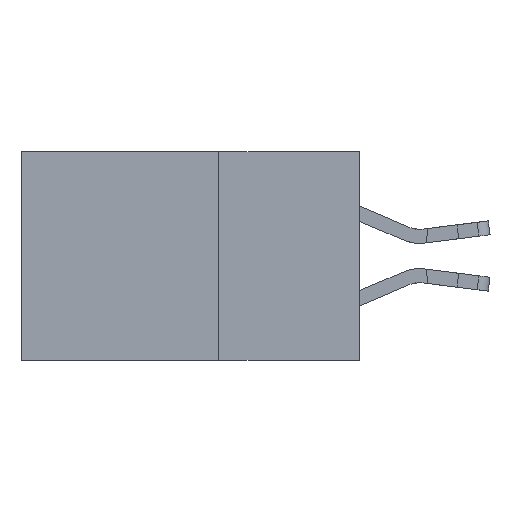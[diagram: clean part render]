
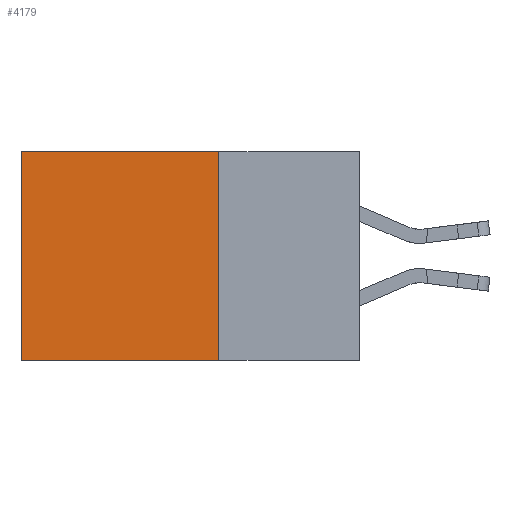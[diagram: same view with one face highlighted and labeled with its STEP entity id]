
A CAD part, left-side view. The second image highlights one B-rep face of the part: STEP entity #4179.
In plain terms, the highlighted planar face has unit normal (-1, 0, 0).
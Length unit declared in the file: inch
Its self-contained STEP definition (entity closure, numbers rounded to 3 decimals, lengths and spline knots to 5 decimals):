
#1412 = CARTESIAN_POINT ( 'NONE',  ( 0.2875, 0.6, 0. ) ) ;
#2165 = EDGE_CURVE ( 'NONE', #9039, #23541, #3738, .T. ) ;
#2648 = FACE_OUTER_BOUND ( 'NONE', #3318, .T. ) ;
#3133 = CARTESIAN_POINT ( 'NONE',  ( 0.2875, 0.6, 0. ) ) ;
#3318 = EDGE_LOOP ( 'NONE', ( #24002, #24450, #4357, #25007 ) ) ;
#3507 = DIRECTION ( 'NONE',  ( 0., 0., -1. ) ) ;
#3738 = LINE ( 'NONE', #13348, #12758 ) ;
#4179 = ADVANCED_FACE ( 'NONE', ( #2648 ), #11461, .F. ) ;
#4357 = ORIENTED_EDGE ( 'NONE', *, *, #16781, .F. ) ;
#6251 = LINE ( 'NONE', #9371, #15902 ) ;
#9039 = VERTEX_POINT ( 'NONE', #24657 ) ;
#9192 = CARTESIAN_POINT ( 'NONE',  ( 0.2875, 0.25, 0. ) ) ;
#9371 = CARTESIAN_POINT ( 'NONE',  ( 0.2875, 0.25, 0. ) ) ;
#9471 = DIRECTION ( 'NONE',  ( 0., 1., 0. ) ) ;
#10163 = EDGE_CURVE ( 'NONE', #23541, #16699, #20910, .T. ) ;
#11364 = DIRECTION ( 'NONE',  ( 0., 0., -1. ) ) ;
#11461 = PLANE ( 'NONE',  #26107 ) ;
#12758 = VECTOR ( 'NONE', #9471, 39.37008 ) ;
#13348 = CARTESIAN_POINT ( 'NONE',  ( 0.2875, 0.25, 0. ) ) ;
#15902 = VECTOR ( 'NONE', #11364, 39.37008 ) ;
#16699 = VERTEX_POINT ( 'NONE', #17055 ) ;
#16781 = EDGE_CURVE ( 'NONE', #9039, #22243, #6251, .T. ) ;
#17055 = CARTESIAN_POINT ( 'NONE',  ( 0.2875, 0.6, -0.37 ) ) ;
#19049 = VECTOR ( 'NONE', #26543, 39.37008 ) ;
#20048 = EDGE_CURVE ( 'NONE', #22243, #16699, #24531, .T. ) ;
#20646 = CARTESIAN_POINT ( 'NONE',  ( 0.2875, 0.25, -0.37 ) ) ;
#20910 = LINE ( 'NONE', #1412, #23823 ) ;
#22243 = VERTEX_POINT ( 'NONE', #24098 ) ;
#23541 = VERTEX_POINT ( 'NONE', #3133 ) ;
#23823 = VECTOR ( 'NONE', #3507, 39.37008 ) ;
#23870 = DIRECTION ( 'NONE',  ( 0., 0., -1. ) ) ;
#24002 = ORIENTED_EDGE ( 'NONE', *, *, #10163, .T. ) ;
#24098 = CARTESIAN_POINT ( 'NONE',  ( 0.2875, 0.25, -0.37 ) ) ;
#24450 = ORIENTED_EDGE ( 'NONE', *, *, #20048, .F. ) ;
#24531 = LINE ( 'NONE', #20646, #19049 ) ;
#24657 = CARTESIAN_POINT ( 'NONE',  ( 0.2875, 0.25, 0. ) ) ;
#25007 = ORIENTED_EDGE ( 'NONE', *, *, #2165, .T. ) ;
#25668 = DIRECTION ( 'NONE',  ( 1., 0., 0. ) ) ;
#26107 = AXIS2_PLACEMENT_3D ( 'NONE', #9192, #25668, #23870 ) ;
#26543 = DIRECTION ( 'NONE',  ( 0., 1., 0. ) ) ;
